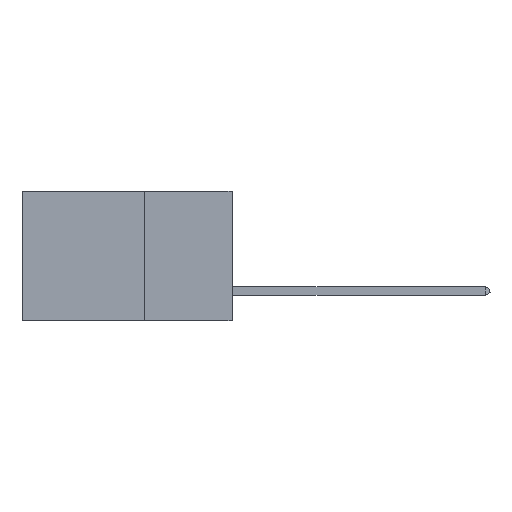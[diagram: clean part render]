
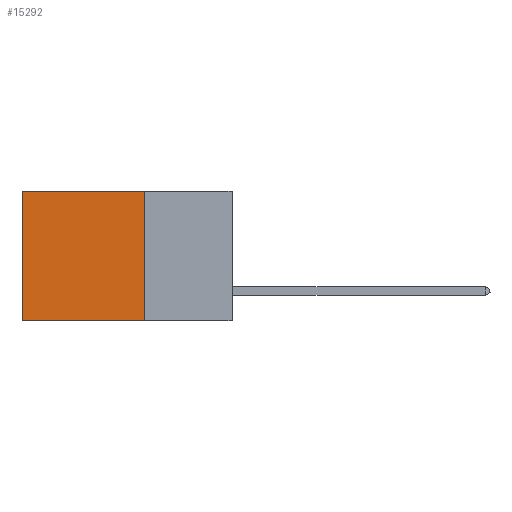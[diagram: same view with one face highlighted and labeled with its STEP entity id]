
A CAD part, left-side view. The second image highlights one B-rep face of the part: STEP entity #15292.
In plain terms, the highlighted planar face has unit normal (-1, 0, 0).
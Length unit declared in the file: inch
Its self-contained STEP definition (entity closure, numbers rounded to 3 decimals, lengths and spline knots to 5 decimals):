
#233 = DIRECTION ( 'NONE',  ( 0., 0., -1. ) ) ;
#543 = ORIENTED_EDGE ( 'NONE', *, *, #5559, .T. ) ;
#580 = VERTEX_POINT ( 'NONE', #11175 ) ;
#919 = DIRECTION ( 'NONE',  ( 1., 0., 0. ) ) ;
#1125 = EDGE_CURVE ( 'NONE', #20141, #14528, #19682, .T. ) ;
#2471 = CARTESIAN_POINT ( 'NONE',  ( 0.2875, 0.25, 0. ) ) ;
#3261 = CARTESIAN_POINT ( 'NONE',  ( 0.2875, 0.25, 0. ) ) ;
#3740 = AXIS2_PLACEMENT_3D ( 'NONE', #2471, #919, #13782 ) ;
#4500 = VERTEX_POINT ( 'NONE', #20254 ) ;
#5559 = EDGE_CURVE ( 'NONE', #4500, #14528, #19816, .T. ) ;
#6700 = CARTESIAN_POINT ( 'NONE',  ( 0.2875, 0.25, -0.37 ) ) ;
#6995 = ORIENTED_EDGE ( 'NONE', *, *, #20270, .F. ) ;
#7196 = VECTOR ( 'NONE', #233, 39.37008 ) ;
#7371 = CARTESIAN_POINT ( 'NONE',  ( 0.2875, 0.6, -0.37 ) ) ;
#7531 = FACE_OUTER_BOUND ( 'NONE', #14780, .T. ) ;
#8009 = DIRECTION ( 'NONE',  ( 0., 0., -1. ) ) ;
#8093 = LINE ( 'NONE', #18974, #14468 ) ;
#8846 = ORIENTED_EDGE ( 'NONE', *, *, #1125, .F. ) ;
#10180 = VECTOR ( 'NONE', #8009, 39.37008 ) ;
#11175 = CARTESIAN_POINT ( 'NONE',  ( 0.2875, 0.25, 0. ) ) ;
#13726 = PLANE ( 'NONE',  #3740 ) ;
#13782 = DIRECTION ( 'NONE',  ( 0., 0., -1. ) ) ;
#14468 = VECTOR ( 'NONE', #20579, 39.37008 ) ;
#14506 = EDGE_CURVE ( 'NONE', #580, #4500, #8093, .T. ) ;
#14528 = VERTEX_POINT ( 'NONE', #7371 ) ;
#14780 = EDGE_LOOP ( 'NONE', ( #543, #8846, #6995, #19680 ) ) ;
#15292 = ADVANCED_FACE ( 'NONE', ( #7531 ), #13726, .F. ) ;
#15816 = CARTESIAN_POINT ( 'NONE',  ( 0.2875, 0.25, -0.37 ) ) ;
#18000 = DIRECTION ( 'NONE',  ( 0., 1., 0. ) ) ;
#18657 = LINE ( 'NONE', #3261, #7196 ) ;
#18974 = CARTESIAN_POINT ( 'NONE',  ( 0.2875, 0.25, 0. ) ) ;
#19680 = ORIENTED_EDGE ( 'NONE', *, *, #14506, .T. ) ;
#19682 = LINE ( 'NONE', #6700, #20413 ) ;
#19816 = LINE ( 'NONE', #21077, #10180 ) ;
#20141 = VERTEX_POINT ( 'NONE', #15816 ) ;
#20254 = CARTESIAN_POINT ( 'NONE',  ( 0.2875, 0.6, 0. ) ) ;
#20270 = EDGE_CURVE ( 'NONE', #580, #20141, #18657, .T. ) ;
#20413 = VECTOR ( 'NONE', #18000, 39.37008 ) ;
#20579 = DIRECTION ( 'NONE',  ( 0., 1., 0. ) ) ;
#21077 = CARTESIAN_POINT ( 'NONE',  ( 0.2875, 0.6, 0. ) ) ;
